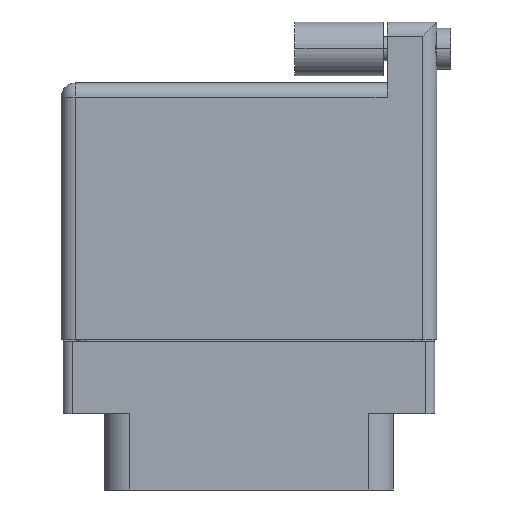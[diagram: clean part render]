
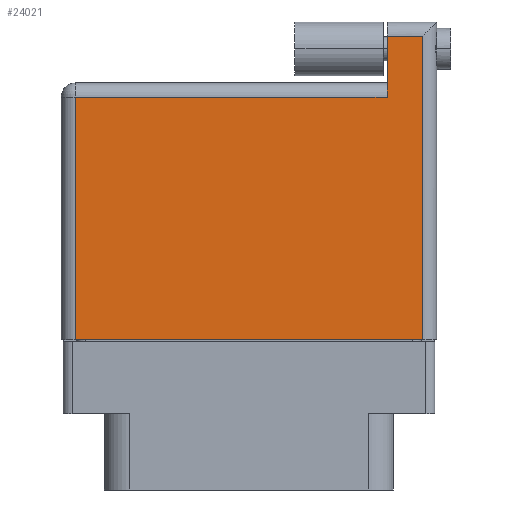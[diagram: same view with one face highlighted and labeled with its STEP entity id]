
A CAD part, front view. The second image highlights one B-rep face of the part: STEP entity #24021.
In plain terms, the highlighted face is planar.
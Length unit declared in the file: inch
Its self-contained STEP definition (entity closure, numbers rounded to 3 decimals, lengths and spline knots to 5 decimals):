
#743 = DIRECTION ( 'NONE',  ( -1., 0., 0. ) ) ;
#846 = EDGE_CURVE ( 'NONE', #18507, #22137, #13321, .T. ) ;
#1549 = DIRECTION ( 'NONE',  ( 0., -1., 0. ) ) ;
#1607 = DIRECTION ( 'NONE',  ( 0., -1., 0. ) ) ;
#3051 = CARTESIAN_POINT ( 'NONE',  ( -0.6625, -0.1, 0.3575 ) ) ;
#3291 = VECTOR ( 'NONE', #20244, 39.37008 ) ;
#4874 = PLANE ( 'NONE',  #16038 ) ;
#5154 = CARTESIAN_POINT ( 'NONE',  ( 0.6125, 0.97, 0.3575 ) ) ;
#5267 = VECTOR ( 'NONE', #1607, 39.37008 ) ;
#6117 = LINE ( 'NONE', #17481, #22773 ) ;
#7571 = LINE ( 'NONE', #12536, #19399 ) ;
#7764 = CARTESIAN_POINT ( 'NONE',  ( -0.6125, -0.1, 0.3575 ) ) ;
#7818 = CARTESIAN_POINT ( 'NONE',  ( -0.6625, 0.97, 0.3575 ) ) ;
#8136 = DIRECTION ( 'NONE',  ( 1., 0., 0. ) ) ;
#8677 = FACE_OUTER_BOUND ( 'NONE', #26425, .T. ) ;
#9430 = CARTESIAN_POINT ( 'NONE',  ( -0.6625, 0.806, 0.3575 ) ) ;
#10036 = EDGE_CURVE ( 'NONE', #27350, #25888, #20837, .T. ) ;
#11943 = ORIENTED_EDGE ( 'NONE', *, *, #20107, .T. ) ;
#12536 = CARTESIAN_POINT ( 'NONE',  ( -0.6625, 0.756, 0.3575 ) ) ;
#13197 = CARTESIAN_POINT ( 'NONE',  ( 0.4875, 0.97, 0.3575 ) ) ;
#13205 = VECTOR ( 'NONE', #26838, 39.37008 ) ;
#13321 = LINE ( 'NONE', #22420, #3291 ) ;
#14083 = DIRECTION ( 'NONE',  ( 0., 0., -1. ) ) ;
#14199 = ORIENTED_EDGE ( 'NONE', *, *, #18870, .T. ) ;
#14819 = EDGE_CURVE ( 'NONE', #29001, #18507, #21204, .T. ) ;
#16038 = AXIS2_PLACEMENT_3D ( 'NONE', #9430, #14083, #23708 ) ;
#16102 = CARTESIAN_POINT ( 'NONE',  ( 0.4875, 1.02, 0.3575 ) ) ;
#17481 = CARTESIAN_POINT ( 'NONE',  ( -0.6125, -0.1, 0.3575 ) ) ;
#18295 = ORIENTED_EDGE ( 'NONE', *, *, #846, .T. ) ;
#18507 = VERTEX_POINT ( 'NONE', #18793 ) ;
#18793 = CARTESIAN_POINT ( 'NONE',  ( 0.6125, -0.1, 0.3575 ) ) ;
#18870 = EDGE_CURVE ( 'NONE', #22137, #27350, #30583, .T. ) ;
#19399 = VECTOR ( 'NONE', #743, 39.37008 ) ;
#20107 = EDGE_CURVE ( 'NONE', #25880, #29001, #6117, .T. ) ;
#20244 = DIRECTION ( 'NONE',  ( 0., 1., 0. ) ) ;
#20837 = LINE ( 'NONE', #16102, #5267 ) ;
#21204 = LINE ( 'NONE', #3051, #29311 ) ;
#22137 = VERTEX_POINT ( 'NONE', #5154 ) ;
#22420 = CARTESIAN_POINT ( 'NONE',  ( 0.6125, 1.02, 0.3575 ) ) ;
#22773 = VECTOR ( 'NONE', #1549, 39.37008 ) ;
#23708 = DIRECTION ( 'NONE',  ( -1., 0., 0. ) ) ;
#23719 = EDGE_CURVE ( 'NONE', #25888, #25880, #7571, .T. ) ;
#24021 = ADVANCED_FACE ( 'NONE', ( #8677 ), #4874, .F. ) ;
#25880 = VERTEX_POINT ( 'NONE', #27889 ) ;
#25888 = VERTEX_POINT ( 'NONE', #27472 ) ;
#26049 = ORIENTED_EDGE ( 'NONE', *, *, #14819, .T. ) ;
#26289 = ORIENTED_EDGE ( 'NONE', *, *, #23719, .T. ) ;
#26425 = EDGE_LOOP ( 'NONE', ( #26049, #18295, #14199, #27268, #26289, #11943 ) ) ;
#26838 = DIRECTION ( 'NONE',  ( -1., 0., 0. ) ) ;
#27268 = ORIENTED_EDGE ( 'NONE', *, *, #10036, .T. ) ;
#27350 = VERTEX_POINT ( 'NONE', #13197 ) ;
#27472 = CARTESIAN_POINT ( 'NONE',  ( 0.4875, 0.756, 0.3575 ) ) ;
#27889 = CARTESIAN_POINT ( 'NONE',  ( -0.6125, 0.756, 0.3575 ) ) ;
#29001 = VERTEX_POINT ( 'NONE', #7764 ) ;
#29311 = VECTOR ( 'NONE', #8136, 39.37008 ) ;
#30583 = LINE ( 'NONE', #7818, #13205 ) ;
